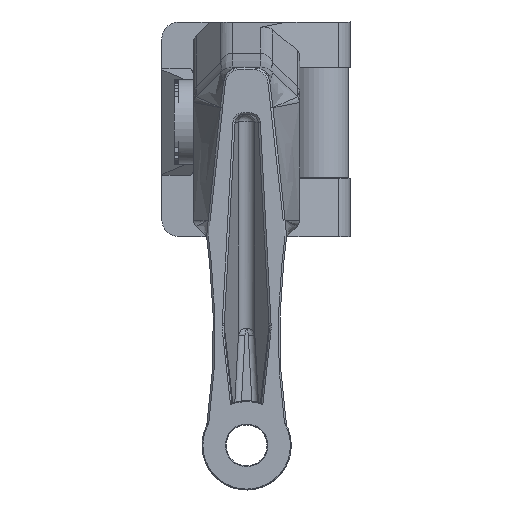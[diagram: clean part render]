
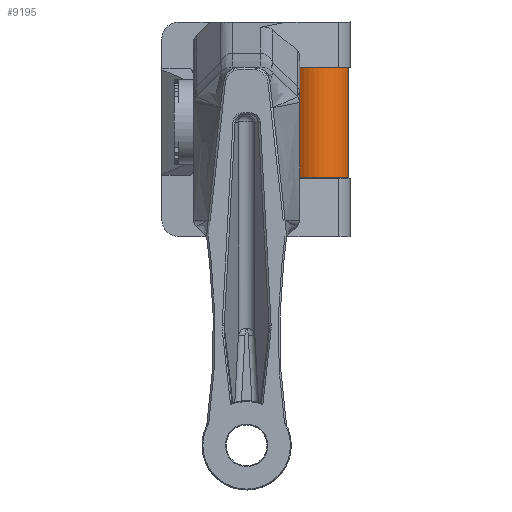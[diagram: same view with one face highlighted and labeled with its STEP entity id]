
A CAD part, left-side view. The second image highlights one B-rep face of the part: STEP entity #9195.
In plain terms, the highlighted cylindrical face has radius 6.9 mm (diameter 13.8 mm), a partial arc.
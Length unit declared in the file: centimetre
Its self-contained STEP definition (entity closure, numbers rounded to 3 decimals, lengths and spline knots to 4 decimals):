
#594=FACE_OUTER_BOUND($,#1182,.T.);
#1182=EDGE_LOOP($,(#6575,#6576,#6577,#6578));
#1821=CIRCLE($,#9778,0.69);
#1834=CIRCLE($,#9811,0.69);
#2205=LINE($,#13576,#3134);
#2240=LINE($,#13669,#3169);
#3134=VECTOR($,#10809,2.59);
#3169=VECTOR($,#10898,2.59);
#4123=VERTEX_POINT($,#13547);
#4124=VERTEX_POINT($,#13549);
#4134=VERTEX_POINT($,#13575);
#4165=VERTEX_POINT($,#13667);
#4981=EDGE_CURVE($,#4124,#4123,#1821,.T.);
#4995=EDGE_CURVE($,#4124,#4134,#2205,.T.);
#5040=EDGE_CURVE($,#4165,#4123,#2240,.T.);
#5041=EDGE_CURVE($,#4165,#4134,#1834,.T.);
#6575=ORIENTED_EDGE($,*,*,#4981,.T.);
#6576=ORIENTED_EDGE($,*,*,#5040,.F.);
#6577=ORIENTED_EDGE($,*,*,#5041,.T.);
#6578=ORIENTED_EDGE($,*,*,#4995,.F.);
#9046=CYLINDRICAL_SURFACE($,#9821,0.69);
#9195=ADVANCED_FACE($,(#594),#9046,.T.);
#9778=AXIS2_PLACEMENT_3D($,#13550,#10788,#10789);
#9811=AXIS2_PLACEMENT_3D($,#13671,#10901,#10902);
#9821=AXIS2_PLACEMENT_3D($,#13691,#10931,#10932);
#10788=DIRECTION('center_axis',(0.,0.,
1.));
#10789=DIRECTION('ref_axis',(0.,-1.,0.));
#10809=DIRECTION($,(0.,0.,1.));
#10898=DIRECTION($,(0.,0.,-1.));
#10901=DIRECTION('center_axis',(0.,0.,
-1.));
#10902=DIRECTION('ref_axis',(0.,-1.,0.));
#10931=DIRECTION('center_axis',(0.,0.,
1.));
#10932=DIRECTION('ref_axis',(0.,-1.,0.));
#13547=CARTESIAN_POINT('',(-11.3744,17.1892,9.076));
#13549=CARTESIAN_POINT('',(-11.3744,18.5692,9.076));
#13550=CARTESIAN_POINT('Origin',(-11.3744,17.8792,9.076));
#13575=CARTESIAN_POINT('',(-11.3744,18.5692,11.666));
#13576=CARTESIAN_POINT($,(-11.3744,18.5692,11.656));
#13667=CARTESIAN_POINT('',(-11.3744,17.1892,11.666));
#13669=CARTESIAN_POINT($,(-11.3744,17.1892,11.656));
#13671=CARTESIAN_POINT('Origin',(-11.3744,17.8792,11.666));
#13691=CARTESIAN_POINT('Origin',(-11.3744,17.8792,11.656));
